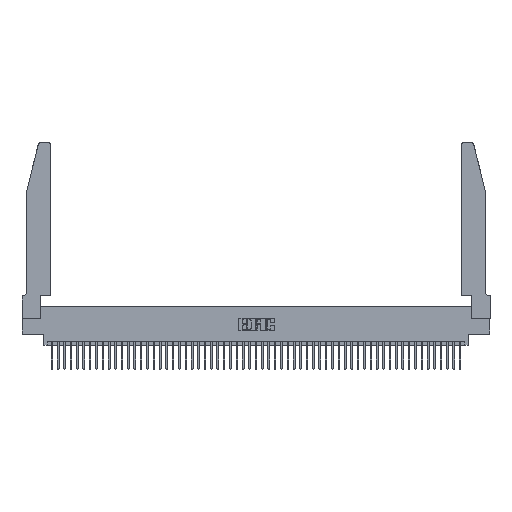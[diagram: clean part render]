
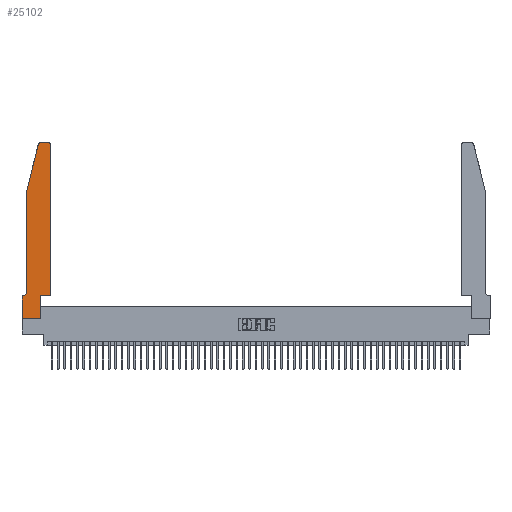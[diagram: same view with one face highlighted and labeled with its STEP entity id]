
A CAD part, top view. The second image highlights one B-rep face of the part: STEP entity #25102.
In plain terms, the highlighted planar face has unit normal (0, 0, 1).
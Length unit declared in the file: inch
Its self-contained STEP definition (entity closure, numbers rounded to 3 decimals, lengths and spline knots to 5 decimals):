
#461 = LINE ( 'NONE', #46994, #42691 ) ;
#520 = DIRECTION ( 'NONE',  ( -0.239, -0.971, 0. ) ) ;
#1013 = VECTOR ( 'NONE', #43754, 39.37008 ) ;
#1055 = CARTESIAN_POINT ( 'NONE',  ( 0.4205, 2.75, 0.37 ) ) ;
#1255 = CIRCLE ( 'NONE', #29903, 0.03 ) ;
#1589 = VECTOR ( 'NONE', #10594, 39.37008 ) ;
#2519 = CARTESIAN_POINT ( 'NONE',  ( 0.2865, 0., 0.37 ) ) ;
#3034 = DIRECTION ( 'NONE',  ( 0., -1., 0. ) ) ;
#3080 = CARTESIAN_POINT ( 'NONE',  ( 0.2605, 2.75, 0.37 ) ) ;
#3322 = ORIENTED_EDGE ( 'NONE', *, *, #32925, .T. ) ;
#3942 = DIRECTION ( 'NONE',  ( 1., 0., 0. ) ) ;
#4679 = CARTESIAN_POINT ( 'NONE',  ( 0.0755, 2., 0.37 ) ) ;
#4805 = CARTESIAN_POINT ( 'NONE',  ( 0., 0.35, 0.37 ) ) ;
#5617 = ORIENTED_EDGE ( 'NONE', *, *, #16394, .T. ) ;
#7535 = LINE ( 'NONE', #51838, #37562 ) ;
#8716 = VERTEX_POINT ( 'NONE', #40722 ) ;
#8814 = CARTESIAN_POINT ( 'NONE',  ( 0.2865, 0.35, 0.37 ) ) ;
#9208 = ORIENTED_EDGE ( 'NONE', *, *, #15292, .T. ) ;
#10224 = CARTESIAN_POINT ( 'NONE',  ( 0.284, 2.72, 0.37 ) ) ;
#10280 = CARTESIAN_POINT ( 'NONE',  ( 0.4205, 2.72, 0.37 ) ) ;
#10594 = DIRECTION ( 'NONE',  ( -1., 0., 0. ) ) ;
#10956 = EDGE_CURVE ( 'NONE', #46030, #31832, #1255, .T. ) ;
#11449 = ORIENTED_EDGE ( 'NONE', *, *, #20694, .T. ) ;
#11561 = VECTOR ( 'NONE', #48591, 39.37008 ) ;
#11653 = CIRCLE ( 'NONE', #43599, 0.07 ) ;
#11965 = CARTESIAN_POINT ( 'NONE',  ( 0.4505, 0.35, 0.37 ) ) ;
#12464 = CARTESIAN_POINT ( 'NONE',  ( 0.4505, 2.72, 0.37 ) ) ;
#12869 = LINE ( 'NONE', #20232, #11561 ) ;
#12960 = DIRECTION ( 'NONE',  ( 0., 1., 0. ) ) ;
#13033 = DIRECTION ( 'NONE',  ( 0., 0., -1. ) ) ;
#13319 = LINE ( 'NONE', #3080, #1013 ) ;
#13627 = ORIENTED_EDGE ( 'NONE', *, *, #36359, .T. ) ;
#13899 = LINE ( 'NONE', #43173, #1589 ) ;
#14372 = DIRECTION ( 'NONE',  ( 1., 0., 0. ) ) ;
#14422 = DIRECTION ( 'NONE',  ( 1., 0., 0. ) ) ;
#15292 = EDGE_CURVE ( 'NONE', #35871, #27068, #461, .T. ) ;
#16394 = EDGE_CURVE ( 'NONE', #31832, #49606, #36234, .T. ) ;
#18267 = VERTEX_POINT ( 'NONE', #12464 ) ;
#19449 = ORIENTED_EDGE ( 'NONE', *, *, #43011, .T. ) ;
#19561 = VERTEX_POINT ( 'NONE', #11965 ) ;
#20072 = EDGE_CURVE ( 'NONE', #27068, #52043, #22320, .T. ) ;
#20232 = CARTESIAN_POINT ( 'NONE',  ( 0.4505, 0.35, 0.37 ) ) ;
#20694 = EDGE_CURVE ( 'NONE', #52043, #52106, #45703, .T. ) ;
#20839 = ORIENTED_EDGE ( 'NONE', *, *, #36919, .T. ) ;
#21408 = CARTESIAN_POINT ( 'NONE',  ( 0., 0., 0.37 ) ) ;
#22256 = CARTESIAN_POINT ( 'NONE',  ( 0.4505, 0.35, 0.37 ) ) ;
#22320 = LINE ( 'NONE', #28036, #42651 ) ;
#23230 = CIRCLE ( 'NONE', #40283, 0.03 ) ;
#24798 = VERTEX_POINT ( 'NONE', #1055 ) ;
#25102 = ADVANCED_FACE ( 'NONE', ( #48823 ), #52747, .T. ) ;
#25328 = ORIENTED_EDGE ( 'NONE', *, *, #10956, .T. ) ;
#27068 = VERTEX_POINT ( 'NONE', #21408 ) ;
#27996 = CARTESIAN_POINT ( 'NONE',  ( 0.0755, 2., 0.37 ) ) ;
#28036 = CARTESIAN_POINT ( 'NONE',  ( 0., 0., 0.37 ) ) ;
#28344 = CARTESIAN_POINT ( 'NONE',  ( 0., 0.35, 0.37 ) ) ;
#28428 = EDGE_CURVE ( 'NONE', #50777, #8716, #11653, .T. ) ;
#28522 = DIRECTION ( 'NONE',  ( 0., 0., 1. ) ) ;
#28711 = EDGE_LOOP ( 'NONE', ( #20839, #25328, #5617, #42700, #36393, #3322, #9208, #33494, #11449, #13627, #39787, #19449 ) ) ;
#29903 = AXIS2_PLACEMENT_3D ( 'NONE', #10224, #38759, #14372 ) ;
#30469 = DIRECTION ( 'NONE',  ( 0., 1., 0. ) ) ;
#30963 = DIRECTION ( 'NONE',  ( 0., -1., 0. ) ) ;
#31832 = VERTEX_POINT ( 'NONE', #52553 ) ;
#32925 = EDGE_CURVE ( 'NONE', #8716, #35871, #13899, .T. ) ;
#33494 = ORIENTED_EDGE ( 'NONE', *, *, #20072, .T. ) ;
#35871 = VERTEX_POINT ( 'NONE', #4805 ) ;
#36091 = CARTESIAN_POINT ( 'NONE',  ( 0.0755, 0.42, 0.37 ) ) ;
#36234 = LINE ( 'NONE', #4679, #45692 ) ;
#36244 = VECTOR ( 'NONE', #12960, 39.37008 ) ;
#36359 = EDGE_CURVE ( 'NONE', #52106, #19561, #12869, .T. ) ;
#36393 = ORIENTED_EDGE ( 'NONE', *, *, #28428, .T. ) ;
#36919 = EDGE_CURVE ( 'NONE', #24798, #46030, #13319, .T. ) ;
#37441 = CARTESIAN_POINT ( 'NONE',  ( 0.284, 2.75, 0.37 ) ) ;
#37455 = CARTESIAN_POINT ( 'NONE',  ( 0.0055, 0.42, 0.37 ) ) ;
#37562 = VECTOR ( 'NONE', #3034, 39.37008 ) ;
#38759 = DIRECTION ( 'NONE',  ( 0., 0., 1. ) ) ;
#38804 = DIRECTION ( 'NONE',  ( 0., 0., 1. ) ) ;
#39787 = ORIENTED_EDGE ( 'NONE', *, *, #40070, .T. ) ;
#40070 = EDGE_CURVE ( 'NONE', #19561, #18267, #45379, .T. ) ;
#40283 = AXIS2_PLACEMENT_3D ( 'NONE', #10280, #38804, #14422 ) ;
#40722 = CARTESIAN_POINT ( 'NONE',  ( 0.0055, 0.35, 0.37 ) ) ;
#41515 = DIRECTION ( 'NONE',  ( -1., 0., 0. ) ) ;
#42651 = VECTOR ( 'NONE', #48196, 39.37008 ) ;
#42691 = VECTOR ( 'NONE', #30963, 39.37008 ) ;
#42700 = ORIENTED_EDGE ( 'NONE', *, *, #52135, .T. ) ;
#42884 = VECTOR ( 'NONE', #30469, 39.37008 ) ;
#43011 = EDGE_CURVE ( 'NONE', #18267, #24798, #23230, .T. ) ;
#43173 = CARTESIAN_POINT ( 'NONE',  ( 0.0755, 0.35, 0.37 ) ) ;
#43559 = CARTESIAN_POINT ( 'NONE',  ( 0.2865, 0.35, 0.37 ) ) ;
#43599 = AXIS2_PLACEMENT_3D ( 'NONE', #37455, #13033, #41515 ) ;
#43754 = DIRECTION ( 'NONE',  ( -1., 0., 0. ) ) ;
#45379 = LINE ( 'NONE', #22256, #42884 ) ;
#45692 = VECTOR ( 'NONE', #520, 39.37008 ) ;
#45703 = LINE ( 'NONE', #8814, #36244 ) ;
#46030 = VERTEX_POINT ( 'NONE', #37441 ) ;
#46520 = AXIS2_PLACEMENT_3D ( 'NONE', #28344, #28522, #3942 ) ;
#46994 = CARTESIAN_POINT ( 'NONE',  ( 0., 0., 0.37 ) ) ;
#48196 = DIRECTION ( 'NONE',  ( 1., 0., 0. ) ) ;
#48591 = DIRECTION ( 'NONE',  ( 1., 0., 0. ) ) ;
#48823 = FACE_OUTER_BOUND ( 'NONE', #28711, .T. ) ;
#49606 = VERTEX_POINT ( 'NONE', #27996 ) ;
#50777 = VERTEX_POINT ( 'NONE', #36091 ) ;
#51838 = CARTESIAN_POINT ( 'NONE',  ( 0.0755, 2., 0.37 ) ) ;
#52043 = VERTEX_POINT ( 'NONE', #2519 ) ;
#52106 = VERTEX_POINT ( 'NONE', #43559 ) ;
#52135 = EDGE_CURVE ( 'NONE', #49606, #50777, #7535, .T. ) ;
#52553 = CARTESIAN_POINT ( 'NONE',  ( 0.25487, 2.72718, 0.37 ) ) ;
#52747 = PLANE ( 'NONE',  #46520 ) ;
